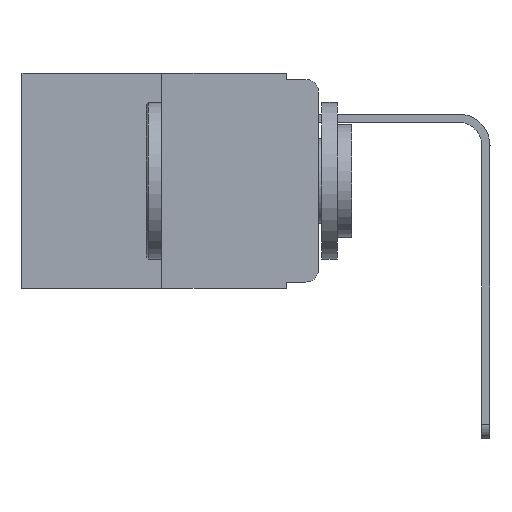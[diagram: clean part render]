
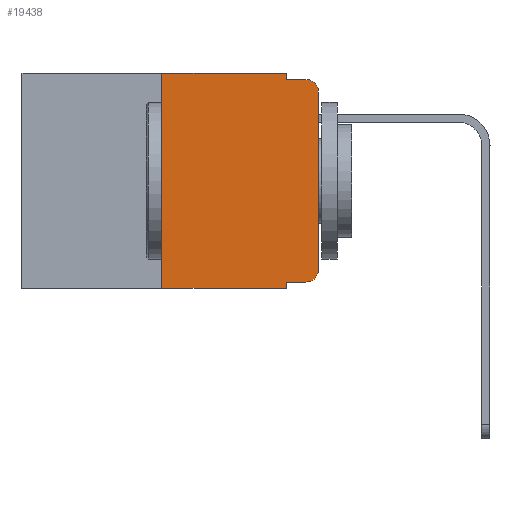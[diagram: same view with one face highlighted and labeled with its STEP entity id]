
A CAD part, left-side view. The second image highlights one B-rep face of the part: STEP entity #19438.
In plain terms, the highlighted planar face has unit normal (-1, 0, 0).
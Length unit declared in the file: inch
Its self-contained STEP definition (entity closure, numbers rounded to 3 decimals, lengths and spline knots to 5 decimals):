
#453 = VECTOR ( 'NONE', #7105, 39.37008 ) ;
#931 = LINE ( 'NONE', #8302, #453 ) ;
#956 = DIRECTION ( 'NONE',  ( 0., 0., 1. ) ) ;
#1013 = CARTESIAN_POINT ( 'NONE',  ( 0., 0., 0. ) ) ;
#1144 = EDGE_CURVE ( 'NONE', #16271, #1231, #4543, .T. ) ;
#1231 = VERTEX_POINT ( 'NONE', #16697 ) ;
#1571 = CARTESIAN_POINT ( 'NONE',  ( 0., 0.051, -0.343 ) ) ;
#1619 = DIRECTION ( 'NONE',  ( 0., -1., 0. ) ) ;
#1823 = CARTESIAN_POINT ( 'NONE',  ( 0., 0.473, 0. ) ) ;
#1904 = EDGE_CURVE ( 'NONE', #13146, #17948, #3543, .T. ) ;
#2010 = DIRECTION ( 'NONE',  ( -1., 0., 0. ) ) ;
#2240 = DIRECTION ( 'NONE',  ( 0., 0., -1. ) ) ;
#2264 = ORIENTED_EDGE ( 'NONE', *, *, #5174, .F. ) ;
#2379 = ORIENTED_EDGE ( 'NONE', *, *, #19168, .T. ) ;
#2662 = ORIENTED_EDGE ( 'NONE', *, *, #1904, .T. ) ;
#2782 = EDGE_CURVE ( 'NONE', #5084, #3389, #16730, .T. ) ;
#3287 = CARTESIAN_POINT ( 'NONE',  ( 0., 0., -0.313 ) ) ;
#3389 = VERTEX_POINT ( 'NONE', #7693 ) ;
#3436 = CARTESIAN_POINT ( 'NONE',  ( 0., 0.25, 0. ) ) ;
#3543 = LINE ( 'NONE', #1013, #15768 ) ;
#3576 = ORIENTED_EDGE ( 'NONE', *, *, #18818, .F. ) ;
#3677 = ORIENTED_EDGE ( 'NONE', *, *, #19196, .T. ) ;
#3888 = VERTEX_POINT ( 'NONE', #10436 ) ;
#4543 = LINE ( 'NONE', #5422, #19976 ) ;
#4632 = ORIENTED_EDGE ( 'NONE', *, *, #2782, .F. ) ;
#4728 = CARTESIAN_POINT ( 'NONE',  ( 0., 0.02, -0.313 ) ) ;
#4871 = DIRECTION ( 'NONE',  ( 0., 0., -1. ) ) ;
#5084 = VERTEX_POINT ( 'NONE', #3436 ) ;
#5174 = EDGE_CURVE ( 'NONE', #3389, #16271, #18729, .T. ) ;
#5251 = AXIS2_PLACEMENT_3D ( 'NONE', #4728, #15675, #4871 ) ;
#5422 = CARTESIAN_POINT ( 'NONE',  ( 0., 0.051, -0.01 ) ) ;
#5444 = LINE ( 'NONE', #15299, #17696 ) ;
#5600 = EDGE_CURVE ( 'NONE', #3888, #19124, #931, .T. ) ;
#5869 = EDGE_LOOP ( 'NONE', ( #2662, #13460, #16089, #2264, #4632, #3576, #3677, #17214, #18609, #2379 ) ) ;
#6143 = LINE ( 'NONE', #17252, #18903 ) ;
#6746 = CARTESIAN_POINT ( 'NONE',  ( 0., 0.02, -0.03 ) ) ;
#6865 = FACE_OUTER_BOUND ( 'NONE', #5869, .T. ) ;
#7105 = DIRECTION ( 'NONE',  ( 0., 0., -1. ) ) ;
#7213 = CARTESIAN_POINT ( 'NONE',  ( 0., 0.25, -0.343 ) ) ;
#7693 = CARTESIAN_POINT ( 'NONE',  ( 0., 0.051, 0. ) ) ;
#8165 = AXIS2_PLACEMENT_3D ( 'NONE', #11614, #14761, #2240 ) ;
#8302 = CARTESIAN_POINT ( 'NONE',  ( 0., 0.051, 0. ) ) ;
#8416 = CARTESIAN_POINT ( 'NONE',  ( 0., 0.02, -0.333 ) ) ;
#10436 = CARTESIAN_POINT ( 'NONE',  ( 0., 0.051, -0.333 ) ) ;
#11527 = CIRCLE ( 'NONE', #13348, 0.02 ) ;
#11530 = VECTOR ( 'NONE', #956, 39.37008 ) ;
#11614 = CARTESIAN_POINT ( 'NONE',  ( 0., 0.473, 0. ) ) ;
#11860 = EDGE_CURVE ( 'NONE', #3888, #14463, #5444, .T. ) ;
#11960 = CARTESIAN_POINT ( 'NONE',  ( 0., 0.25, 0. ) ) ;
#12284 = DIRECTION ( 'NONE',  ( 0., -1., 0. ) ) ;
#13016 = DIRECTION ( 'NONE',  ( 0., 0., -1. ) ) ;
#13146 = VERTEX_POINT ( 'NONE', #3287 ) ;
#13348 = AXIS2_PLACEMENT_3D ( 'NONE', #6746, #2010, #13016 ) ;
#13460 = ORIENTED_EDGE ( 'NONE', *, *, #18216, .T. ) ;
#13670 = VECTOR ( 'NONE', #18459, 39.37008 ) ;
#13990 = CARTESIAN_POINT ( 'NONE',  ( 0., 0., -0.03 ) ) ;
#14161 = DIRECTION ( 'NONE',  ( 0., -1., 0. ) ) ;
#14229 = VERTEX_POINT ( 'NONE', #7213 ) ;
#14463 = VERTEX_POINT ( 'NONE', #8416 ) ;
#14761 = DIRECTION ( 'NONE',  ( 1., 0., 0. ) ) ;
#14825 = PLANE ( 'NONE',  #8165 ) ;
#15216 = CARTESIAN_POINT ( 'NONE',  ( 0., 0.051, 0. ) ) ;
#15299 = CARTESIAN_POINT ( 'NONE',  ( 0., 0.051, -0.333 ) ) ;
#15675 = DIRECTION ( 'NONE',  ( -1., 0., 0. ) ) ;
#15705 = LINE ( 'NONE', #11960, #11530 ) ;
#15768 = VECTOR ( 'NONE', #18086, 39.37008 ) ;
#16089 = ORIENTED_EDGE ( 'NONE', *, *, #1144, .F. ) ;
#16271 = VERTEX_POINT ( 'NONE', #18404 ) ;
#16697 = CARTESIAN_POINT ( 'NONE',  ( 0., 0.02, -0.01 ) ) ;
#16730 = LINE ( 'NONE', #1823, #18212 ) ;
#17214 = ORIENTED_EDGE ( 'NONE', *, *, #5600, .F. ) ;
#17252 = CARTESIAN_POINT ( 'NONE',  ( 0., 0.473, -0.343 ) ) ;
#17696 = VECTOR ( 'NONE', #12284, 39.37008 ) ;
#17948 = VERTEX_POINT ( 'NONE', #13990 ) ;
#18086 = DIRECTION ( 'NONE',  ( 0., 0., 1. ) ) ;
#18212 = VECTOR ( 'NONE', #1619, 39.37008 ) ;
#18216 = EDGE_CURVE ( 'NONE', #17948, #1231, #11527, .T. ) ;
#18404 = CARTESIAN_POINT ( 'NONE',  ( 0., 0.051, -0.01 ) ) ;
#18459 = DIRECTION ( 'NONE',  ( 0., 0., -1. ) ) ;
#18609 = ORIENTED_EDGE ( 'NONE', *, *, #11860, .T. ) ;
#18729 = LINE ( 'NONE', #15216, #13670 ) ;
#18818 = EDGE_CURVE ( 'NONE', #14229, #5084, #15705, .T. ) ;
#18903 = VECTOR ( 'NONE', #14161, 39.37008 ) ;
#19124 = VERTEX_POINT ( 'NONE', #1571 ) ;
#19168 = EDGE_CURVE ( 'NONE', #14463, #13146, #20104, .T. ) ;
#19196 = EDGE_CURVE ( 'NONE', #14229, #19124, #6143, .T. ) ;
#19438 = ADVANCED_FACE ( 'NONE', ( #6865 ), #14825, .F. ) ;
#19657 = DIRECTION ( 'NONE',  ( 0., -1., 0. ) ) ;
#19976 = VECTOR ( 'NONE', #19657, 39.37008 ) ;
#20104 = CIRCLE ( 'NONE', #5251, 0.02 ) ;
